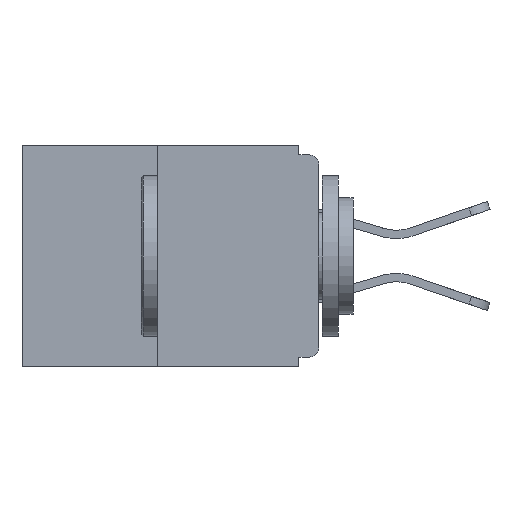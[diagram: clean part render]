
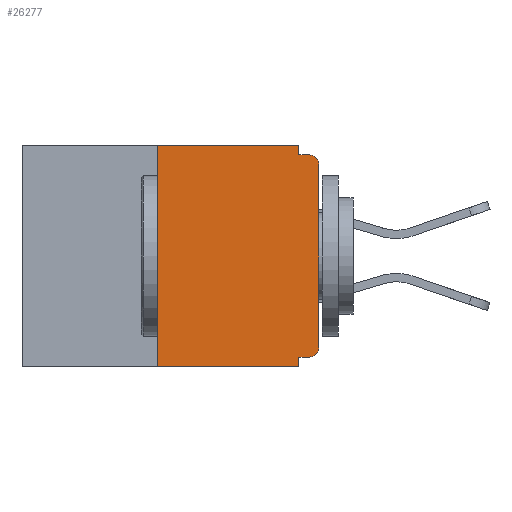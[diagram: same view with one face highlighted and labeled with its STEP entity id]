
A CAD part, left-side view. The second image highlights one B-rep face of the part: STEP entity #26277.
In plain terms, the highlighted planar face has unit normal (-1, 0, 0).
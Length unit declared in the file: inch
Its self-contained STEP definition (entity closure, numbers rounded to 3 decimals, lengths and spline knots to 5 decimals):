
#116 = CARTESIAN_POINT ( 'NONE',  ( 0., 0.46, 0. ) ) ;
#413 = FACE_OUTER_BOUND ( 'NONE', #1338, .T. ) ;
#676 = DIRECTION ( 'NONE',  ( -1., 0., 0. ) ) ;
#1107 = DIRECTION ( 'NONE',  ( 0., -1., 0. ) ) ;
#1338 = EDGE_LOOP ( 'NONE', ( #3472, #20316, #22597, #29213, #6492, #3460, #18359, #15939, #23171, #2016 ) ) ;
#2016 = ORIENTED_EDGE ( 'NONE', *, *, #15308, .F. ) ;
#2040 = LINE ( 'NONE', #27902, #12869 ) ;
#2470 = AXIS2_PLACEMENT_3D ( 'NONE', #12190, #676, #28095 ) ;
#2672 = LINE ( 'NONE', #11658, #16417 ) ;
#2772 = CARTESIAN_POINT ( 'NONE',  ( 0., 0.46, 0. ) ) ;
#3460 = ORIENTED_EDGE ( 'NONE', *, *, #15436, .T. ) ;
#3469 = EDGE_CURVE ( 'NONE', #6387, #20975, #29442, .T. ) ;
#3472 = ORIENTED_EDGE ( 'NONE', *, *, #12623, .F. ) ;
#3811 = CARTESIAN_POINT ( 'NONE',  ( 0., 0., -0.328 ) ) ;
#3910 = CARTESIAN_POINT ( 'NONE',  ( 0., 0.25, 0. ) ) ;
#5075 = EDGE_CURVE ( 'NONE', #25255, #7245, #2672, .T. ) ;
#5656 = CARTESIAN_POINT ( 'NONE',  ( 0., 0., -0.03 ) ) ;
#6034 = EDGE_CURVE ( 'NONE', #14588, #10829, #29660, .T. ) ;
#6254 = DIRECTION ( 'NONE',  ( 0., 0., 1. ) ) ;
#6387 = VERTEX_POINT ( 'NONE', #9679 ) ;
#6492 = ORIENTED_EDGE ( 'NONE', *, *, #6034, .F. ) ;
#6612 = EDGE_CURVE ( 'NONE', #10829, #11610, #25651, .T. ) ;
#7116 = CIRCLE ( 'NONE', #2470, 0.015 ) ;
#7245 = VERTEX_POINT ( 'NONE', #5656 ) ;
#7285 = VECTOR ( 'NONE', #15683, 39.37008 ) ;
#7310 = PLANE ( 'NONE',  #9638 ) ;
#9531 = DIRECTION ( 'NONE',  ( 1., 0., 0. ) ) ;
#9638 = AXIS2_PLACEMENT_3D ( 'NONE', #116, #9531, #25622 ) ;
#9679 = CARTESIAN_POINT ( 'NONE',  ( 0., 0.25, -0.343 ) ) ;
#9754 = DIRECTION ( 'NONE',  ( 0., -1., 0. ) ) ;
#10346 = AXIS2_PLACEMENT_3D ( 'NONE', #27941, #14288, #25422 ) ;
#10390 = CARTESIAN_POINT ( 'NONE',  ( 0., 0.031, 0. ) ) ;
#10580 = VECTOR ( 'NONE', #10905, 39.37008 ) ;
#10583 = VECTOR ( 'NONE', #1107, 39.37008 ) ;
#10671 = CARTESIAN_POINT ( 'NONE',  ( 0., 0., -0.313 ) ) ;
#10829 = VERTEX_POINT ( 'NONE', #21138 ) ;
#10905 = DIRECTION ( 'NONE',  ( 0., 1., 0. ) ) ;
#11610 = VERTEX_POINT ( 'NONE', #16971 ) ;
#11658 = CARTESIAN_POINT ( 'NONE',  ( 0., 0., 0. ) ) ;
#12190 = CARTESIAN_POINT ( 'NONE',  ( 0., 0.015, -0.313 ) ) ;
#12623 = EDGE_CURVE ( 'NONE', #20975, #25132, #19247, .T. ) ;
#12869 = VECTOR ( 'NONE', #22971, 39.37008 ) ;
#13346 = CARTESIAN_POINT ( 'NONE',  ( 0., 0.031, -0.343 ) ) ;
#13993 = VECTOR ( 'NONE', #6254, 39.37008 ) ;
#14288 = DIRECTION ( 'NONE',  ( -1., 0., 0. ) ) ;
#14588 = VERTEX_POINT ( 'NONE', #24704 ) ;
#15308 = EDGE_CURVE ( 'NONE', #25132, #27134, #2040, .T. ) ;
#15436 = EDGE_CURVE ( 'NONE', #14588, #25255, #7116, .T. ) ;
#15683 = DIRECTION ( 'NONE',  ( 0., 0., -1. ) ) ;
#15939 = ORIENTED_EDGE ( 'NONE', *, *, #23401, .T. ) ;
#16417 = VECTOR ( 'NONE', #20931, 39.37008 ) ;
#16971 = CARTESIAN_POINT ( 'NONE',  ( 0., 0.031, -0.343 ) ) ;
#18359 = ORIENTED_EDGE ( 'NONE', *, *, #5075, .T. ) ;
#18520 = LINE ( 'NONE', #19768, #10583 ) ;
#19247 = LINE ( 'NONE', #2772, #24606 ) ;
#19373 = VECTOR ( 'NONE', #23157, 39.37008 ) ;
#19576 = EDGE_CURVE ( 'NONE', #27134, #29242, #18520, .T. ) ;
#19768 = CARTESIAN_POINT ( 'NONE',  ( 0., 0., -0.015 ) ) ;
#20316 = ORIENTED_EDGE ( 'NONE', *, *, #3469, .F. ) ;
#20931 = DIRECTION ( 'NONE',  ( 0., 0., 1. ) ) ;
#20975 = VERTEX_POINT ( 'NONE', #27022 ) ;
#21118 = CARTESIAN_POINT ( 'NONE',  ( 0., 0.015, -0.015 ) ) ;
#21138 = CARTESIAN_POINT ( 'NONE',  ( 0., 0.031, -0.328 ) ) ;
#22597 = ORIENTED_EDGE ( 'NONE', *, *, #22857, .T. ) ;
#22857 = EDGE_CURVE ( 'NONE', #6387, #11610, #25466, .T. ) ;
#22971 = DIRECTION ( 'NONE',  ( 0., 0., -1. ) ) ;
#23157 = DIRECTION ( 'NONE',  ( 0., -1., 0. ) ) ;
#23171 = ORIENTED_EDGE ( 'NONE', *, *, #19576, .F. ) ;
#23401 = EDGE_CURVE ( 'NONE', #7245, #29242, #24343, .T. ) ;
#24343 = CIRCLE ( 'NONE', #10346, 0.015 ) ;
#24606 = VECTOR ( 'NONE', #9754, 39.37008 ) ;
#24704 = CARTESIAN_POINT ( 'NONE',  ( 0., 0.015, -0.328 ) ) ;
#24849 = CARTESIAN_POINT ( 'NONE',  ( 0., 0.031, -0.015 ) ) ;
#25132 = VERTEX_POINT ( 'NONE', #10390 ) ;
#25255 = VERTEX_POINT ( 'NONE', #10671 ) ;
#25422 = DIRECTION ( 'NONE',  ( 0., 0., -1. ) ) ;
#25466 = LINE ( 'NONE', #27962, #19373 ) ;
#25622 = DIRECTION ( 'NONE',  ( 0., 0., -1. ) ) ;
#25651 = LINE ( 'NONE', #13346, #7285 ) ;
#26277 = ADVANCED_FACE ( 'NONE', ( #413 ), #7310, .F. ) ;
#27022 = CARTESIAN_POINT ( 'NONE',  ( 0., 0.25, 0. ) ) ;
#27134 = VERTEX_POINT ( 'NONE', #24849 ) ;
#27902 = CARTESIAN_POINT ( 'NONE',  ( 0., 0.031, 0. ) ) ;
#27941 = CARTESIAN_POINT ( 'NONE',  ( 0., 0.015, -0.03 ) ) ;
#27962 = CARTESIAN_POINT ( 'NONE',  ( 0., 0.46, -0.343 ) ) ;
#28095 = DIRECTION ( 'NONE',  ( 0., 0., -1. ) ) ;
#29213 = ORIENTED_EDGE ( 'NONE', *, *, #6612, .F. ) ;
#29242 = VERTEX_POINT ( 'NONE', #21118 ) ;
#29442 = LINE ( 'NONE', #3910, #13993 ) ;
#29660 = LINE ( 'NONE', #3811, #10580 ) ;
